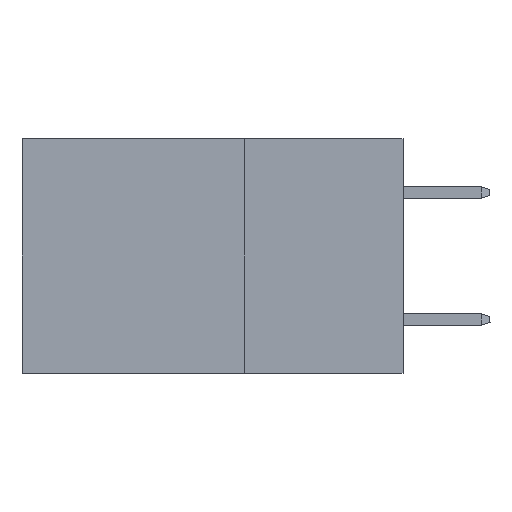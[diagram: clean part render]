
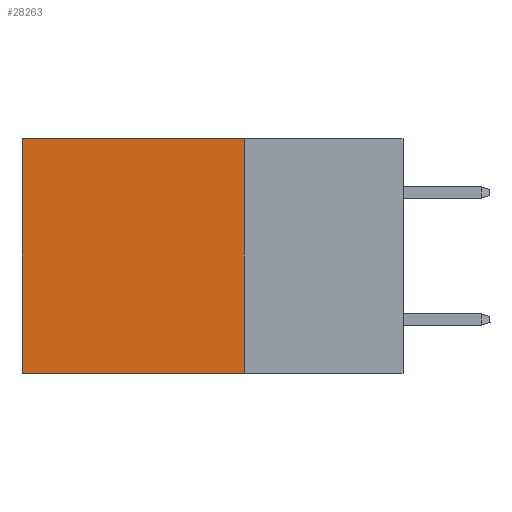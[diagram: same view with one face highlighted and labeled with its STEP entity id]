
A CAD part, left-side view. The second image highlights one B-rep face of the part: STEP entity #28263.
In plain terms, the highlighted planar face has unit normal (-1, 0, 0).
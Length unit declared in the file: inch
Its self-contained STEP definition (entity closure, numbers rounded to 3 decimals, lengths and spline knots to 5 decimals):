
#346 = AXIS2_PLACEMENT_3D ( 'NONE', #22546, #27530, #6849 ) ;
#565 = EDGE_CURVE ( 'NONE', #27668, #19608, #7972, .T. ) ;
#566 = EDGE_LOOP ( 'NONE', ( #1362, #27728, #3278, #18489 ) ) ;
#674 = FACE_OUTER_BOUND ( 'NONE', #566, .T. ) ;
#1362 = ORIENTED_EDGE ( 'NONE', *, *, #565, .T. ) ;
#2168 = DIRECTION ( 'NONE',  ( 0., 0., -1. ) ) ;
#3278 = ORIENTED_EDGE ( 'NONE', *, *, #14248, .F. ) ;
#4330 = CARTESIAN_POINT ( 'NONE',  ( 0.2875, 0.6, -0.37 ) ) ;
#6849 = DIRECTION ( 'NONE',  ( 0., 0., -1. ) ) ;
#7176 = LINE ( 'NONE', #12629, #15599 ) ;
#7767 = LINE ( 'NONE', #29795, #7803 ) ;
#7803 = VECTOR ( 'NONE', #15149, 39.37008 ) ;
#7972 = LINE ( 'NONE', #22913, #24373 ) ;
#11880 = VERTEX_POINT ( 'NONE', #19108 ) ;
#11992 = VECTOR ( 'NONE', #22235, 39.37008 ) ;
#12273 = CARTESIAN_POINT ( 'NONE',  ( 0.2875, 0.25, -0.37 ) ) ;
#12493 = EDGE_CURVE ( 'NONE', #15109, #27668, #7767, .T. ) ;
#12629 = CARTESIAN_POINT ( 'NONE',  ( 0.2875, 0.25, 0. ) ) ;
#14248 = EDGE_CURVE ( 'NONE', #15109, #11880, #7176, .T. ) ;
#15109 = VERTEX_POINT ( 'NONE', #30744 ) ;
#15149 = DIRECTION ( 'NONE',  ( 0., 1., 0. ) ) ;
#15599 = VECTOR ( 'NONE', #2168, 39.37008 ) ;
#16165 = EDGE_CURVE ( 'NONE', #11880, #19608, #22076, .T. ) ;
#16517 = CARTESIAN_POINT ( 'NONE',  ( 0.2875, 0.6, 0. ) ) ;
#17718 = PLANE ( 'NONE',  #346 ) ;
#18489 = ORIENTED_EDGE ( 'NONE', *, *, #12493, .T. ) ;
#19108 = CARTESIAN_POINT ( 'NONE',  ( 0.2875, 0.25, -0.37 ) ) ;
#19608 = VERTEX_POINT ( 'NONE', #4330 ) ;
#22076 = LINE ( 'NONE', #12273, #11992 ) ;
#22235 = DIRECTION ( 'NONE',  ( 0., 1., 0. ) ) ;
#22546 = CARTESIAN_POINT ( 'NONE',  ( 0.2875, 0.25, 0. ) ) ;
#22760 = DIRECTION ( 'NONE',  ( 0., 0., -1. ) ) ;
#22913 = CARTESIAN_POINT ( 'NONE',  ( 0.2875, 0.6, 0. ) ) ;
#24373 = VECTOR ( 'NONE', #22760, 39.37008 ) ;
#27530 = DIRECTION ( 'NONE',  ( 1., 0., 0. ) ) ;
#27668 = VERTEX_POINT ( 'NONE', #16517 ) ;
#27728 = ORIENTED_EDGE ( 'NONE', *, *, #16165, .F. ) ;
#28263 = ADVANCED_FACE ( 'NONE', ( #674 ), #17718, .F. ) ;
#29795 = CARTESIAN_POINT ( 'NONE',  ( 0.2875, 0.25, 0. ) ) ;
#30744 = CARTESIAN_POINT ( 'NONE',  ( 0.2875, 0.25, 0. ) ) ;
